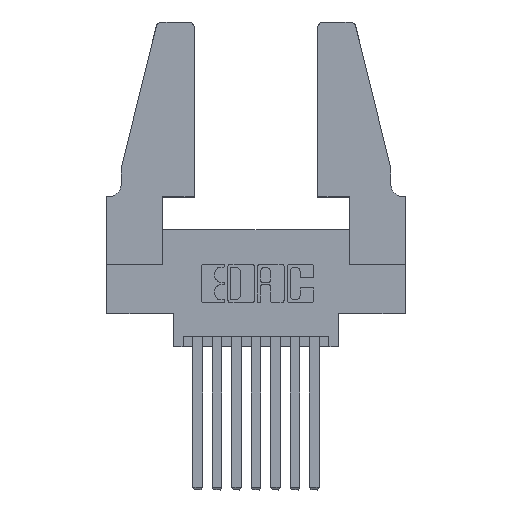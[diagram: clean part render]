
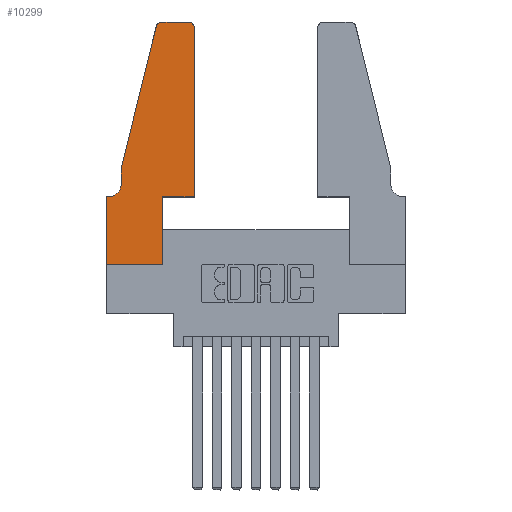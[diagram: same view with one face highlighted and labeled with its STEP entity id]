
A CAD part, top view. The second image highlights one B-rep face of the part: STEP entity #10299.
In plain terms, the highlighted planar face has unit normal (0, 0, 1).
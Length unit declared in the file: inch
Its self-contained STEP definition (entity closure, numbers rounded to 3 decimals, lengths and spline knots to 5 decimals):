
#155 = CIRCLE ( 'NONE', #10700, 0.07 ) ;
#249 = EDGE_CURVE ( 'NONE', #6374, #12025, #155, .T. ) ;
#261 = CIRCLE ( 'NONE', #909, 0.03 ) ;
#313 = VERTEX_POINT ( 'NONE', #11717 ) ;
#407 = EDGE_CURVE ( 'NONE', #880, #7144, #6180, .T. ) ;
#435 = VERTEX_POINT ( 'NONE', #4326 ) ;
#484 = DIRECTION ( 'NONE',  ( 1., 0., 0. ) ) ;
#504 = ORIENTED_EDGE ( 'NONE', *, *, #1265, .T. ) ;
#640 = LINE ( 'NONE', #11129, #10147 ) ;
#839 = DIRECTION ( 'NONE',  ( -1., 0., 0. ) ) ;
#880 = VERTEX_POINT ( 'NONE', #5089 ) ;
#909 = AXIS2_PLACEMENT_3D ( 'NONE', #3608, #10101, #4605 ) ;
#1265 = EDGE_CURVE ( 'NONE', #313, #9736, #11399, .T. ) ;
#1390 = VECTOR ( 'NONE', #7709, 39.37008 ) ;
#1732 = VERTEX_POINT ( 'NONE', #4247 ) ;
#2383 = ORIENTED_EDGE ( 'NONE', *, *, #249, .T. ) ;
#2786 = DIRECTION ( 'NONE',  ( -1., 0., 0. ) ) ;
#2815 = DIRECTION ( 'NONE',  ( -1., 0., 0. ) ) ;
#3048 = CARTESIAN_POINT ( 'NONE',  ( 0.2605, 1.25, 0.37 ) ) ;
#3460 = AXIS2_PLACEMENT_3D ( 'NONE', #11115, #11152, #5664 ) ;
#3608 = CARTESIAN_POINT ( 'NONE',  ( 0.4205, 1.22, 0.37 ) ) ;
#3659 = EDGE_CURVE ( 'NONE', #8053, #880, #4857, .T. ) ;
#3925 = CARTESIAN_POINT ( 'NONE',  ( 0.2865, 0.35, 0.37 ) ) ;
#4095 = VECTOR ( 'NONE', #8606, 39.37008 ) ;
#4148 = ORIENTED_EDGE ( 'NONE', *, *, #4306, .T. ) ;
#4247 = CARTESIAN_POINT ( 'NONE',  ( 0.2865, 0., 0.37 ) ) ;
#4306 = EDGE_CURVE ( 'NONE', #11393, #6374, #640, .T. ) ;
#4326 = CARTESIAN_POINT ( 'NONE',  ( 0., 0.35, 0.37 ) ) ;
#4542 = CARTESIAN_POINT ( 'NONE',  ( 0., 0., 0.37 ) ) ;
#4605 = DIRECTION ( 'NONE',  ( 1., 0., 0. ) ) ;
#4606 = CARTESIAN_POINT ( 'NONE',  ( 0.4505, 0.35, 0.37 ) ) ;
#4857 = LINE ( 'NONE', #7742, #9457 ) ;
#4911 = VECTOR ( 'NONE', #2786, 39.37008 ) ;
#4913 = CARTESIAN_POINT ( 'NONE',  ( 0.4505, 1.22, 0.37 ) ) ;
#5089 = CARTESIAN_POINT ( 'NONE',  ( 0.4505, 0.35, 0.37 ) ) ;
#5379 = DIRECTION ( 'NONE',  ( 0., 1., 0. ) ) ;
#5664 = DIRECTION ( 'NONE',  ( 1., 0., 0. ) ) ;
#5802 = DIRECTION ( 'NONE',  ( 0., 0., -1. ) ) ;
#5937 = ORIENTED_EDGE ( 'NONE', *, *, #6270, .T. ) ;
#6180 = LINE ( 'NONE', #4606, #6471 ) ;
#6270 = EDGE_CURVE ( 'NONE', #9736, #6856, #10696, .T. ) ;
#6350 = EDGE_CURVE ( 'NONE', #7144, #313, #261, .T. ) ;
#6355 = DIRECTION ( 'NONE',  ( 0., 0., 1. ) ) ;
#6374 = VERTEX_POINT ( 'NONE', #9196 ) ;
#6471 = VECTOR ( 'NONE', #5379, 39.37008 ) ;
#6613 = LINE ( 'NONE', #3925, #4095 ) ;
#6670 = VECTOR ( 'NONE', #10038, 39.37008 ) ;
#6806 = CARTESIAN_POINT ( 'NONE',  ( 0.0755, 0.5, 0.37 ) ) ;
#6856 = VERTEX_POINT ( 'NONE', #8250 ) ;
#6952 = LINE ( 'NONE', #4542, #6670 ) ;
#7041 = FACE_OUTER_BOUND ( 'NONE', #11209, .T. ) ;
#7144 = VERTEX_POINT ( 'NONE', #4913 ) ;
#7414 = VERTEX_POINT ( 'NONE', #9046 ) ;
#7465 = EDGE_CURVE ( 'NONE', #435, #7414, #6952, .T. ) ;
#7705 = EDGE_CURVE ( 'NONE', #6856, #11393, #11429, .T. ) ;
#7709 = DIRECTION ( 'NONE',  ( -0.239, -0.971, 0. ) ) ;
#7742 = CARTESIAN_POINT ( 'NONE',  ( 0.4505, 0.35, 0.37 ) ) ;
#7899 = DIRECTION ( 'NONE',  ( 1., 0., 0. ) ) ;
#8053 = VERTEX_POINT ( 'NONE', #9075 ) ;
#8073 = ORIENTED_EDGE ( 'NONE', *, *, #8149, .T. ) ;
#8149 = EDGE_CURVE ( 'NONE', #7414, #1732, #11716, .T. ) ;
#8250 = CARTESIAN_POINT ( 'NONE',  ( 0.25487, 1.22718, 0.37 ) ) ;
#8369 = PLANE ( 'NONE',  #3460 ) ;
#8508 = ORIENTED_EDGE ( 'NONE', *, *, #407, .T. ) ;
#8564 = ORIENTED_EDGE ( 'NONE', *, *, #8628, .T. ) ;
#8606 = DIRECTION ( 'NONE',  ( 0., 1., 0. ) ) ;
#8628 = EDGE_CURVE ( 'NONE', #12025, #435, #11705, .T. ) ;
#8631 = ORIENTED_EDGE ( 'NONE', *, *, #6350, .T. ) ;
#8660 = VECTOR ( 'NONE', #839, 39.37008 ) ;
#8672 = ORIENTED_EDGE ( 'NONE', *, *, #7705, .T. ) ;
#8959 = VECTOR ( 'NONE', #10142, 39.37008 ) ;
#9046 = CARTESIAN_POINT ( 'NONE',  ( 0., 0., 0.37 ) ) ;
#9075 = CARTESIAN_POINT ( 'NONE',  ( 0.2865, 0.35, 0.37 ) ) ;
#9112 = CARTESIAN_POINT ( 'NONE',  ( 0.0755, 0.5, 0.37 ) ) ;
#9189 = CARTESIAN_POINT ( 'NONE',  ( 0.0055, 0.35, 0.37 ) ) ;
#9196 = CARTESIAN_POINT ( 'NONE',  ( 0.0755, 0.42, 0.37 ) ) ;
#9357 = CARTESIAN_POINT ( 'NONE',  ( 0.284, 1.25, 0.37 ) ) ;
#9457 = VECTOR ( 'NONE', #7899, 39.37008 ) ;
#9736 = VERTEX_POINT ( 'NONE', #9357 ) ;
#10038 = DIRECTION ( 'NONE',  ( 0., -1., 0. ) ) ;
#10101 = DIRECTION ( 'NONE',  ( 0., 0., 1. ) ) ;
#10142 = DIRECTION ( 'NONE',  ( 1., 0., 0. ) ) ;
#10147 = VECTOR ( 'NONE', #11008, 39.37008 ) ;
#10299 = ADVANCED_FACE ( 'NONE', ( #7041 ), #8369, .T. ) ;
#10347 = ORIENTED_EDGE ( 'NONE', *, *, #7465, .T. ) ;
#10660 = AXIS2_PLACEMENT_3D ( 'NONE', #11861, #6355, #484 ) ;
#10696 = CIRCLE ( 'NONE', #10660, 0.03 ) ;
#10700 = AXIS2_PLACEMENT_3D ( 'NONE', #11353, #5802, #2815 ) ;
#11008 = DIRECTION ( 'NONE',  ( 0., -1., 0. ) ) ;
#11029 = EDGE_CURVE ( 'NONE', #1732, #8053, #6613, .T. ) ;
#11052 = CARTESIAN_POINT ( 'NONE',  ( 0., 0., 0.37 ) ) ;
#11115 = CARTESIAN_POINT ( 'NONE',  ( 0., 0.35, 0.37 ) ) ;
#11129 = CARTESIAN_POINT ( 'NONE',  ( 0.0755, 0.5, 0.37 ) ) ;
#11152 = DIRECTION ( 'NONE',  ( 0., 0., 1. ) ) ;
#11209 = EDGE_LOOP ( 'NONE', ( #504, #5937, #8672, #4148, #2383, #8564, #10347, #8073, #11638, #12123, #8508, #8631 ) ) ;
#11353 = CARTESIAN_POINT ( 'NONE',  ( 0.0055, 0.42, 0.37 ) ) ;
#11393 = VERTEX_POINT ( 'NONE', #9112 ) ;
#11399 = LINE ( 'NONE', #3048, #4911 ) ;
#11429 = LINE ( 'NONE', #6806, #1390 ) ;
#11638 = ORIENTED_EDGE ( 'NONE', *, *, #11029, .T. ) ;
#11705 = LINE ( 'NONE', #12137, #8660 ) ;
#11716 = LINE ( 'NONE', #11052, #8959 ) ;
#11717 = CARTESIAN_POINT ( 'NONE',  ( 0.4205, 1.25, 0.37 ) ) ;
#11861 = CARTESIAN_POINT ( 'NONE',  ( 0.284, 1.22, 0.37 ) ) ;
#12025 = VERTEX_POINT ( 'NONE', #9189 ) ;
#12123 = ORIENTED_EDGE ( 'NONE', *, *, #3659, .T. ) ;
#12137 = CARTESIAN_POINT ( 'NONE',  ( 0.0755, 0.35, 0.37 ) ) ;
